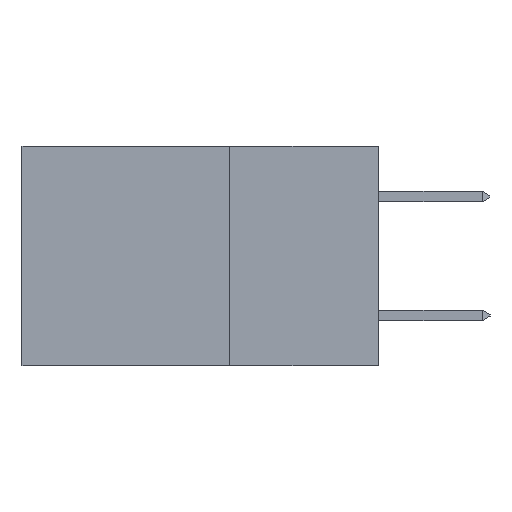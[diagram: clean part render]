
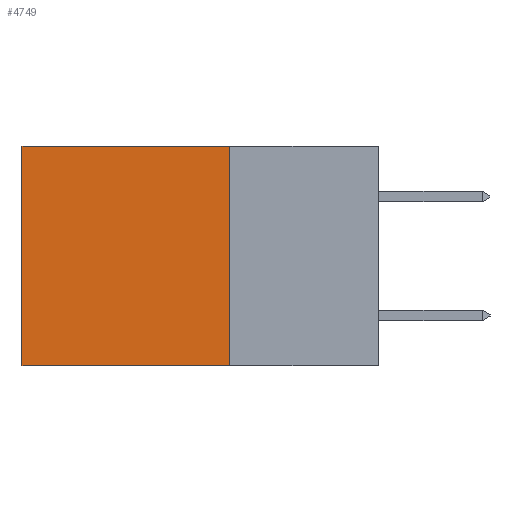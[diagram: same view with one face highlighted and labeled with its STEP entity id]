
A CAD part, left-side view. The second image highlights one B-rep face of the part: STEP entity #4749.
In plain terms, the highlighted planar face has unit normal (-1, 0, 0).
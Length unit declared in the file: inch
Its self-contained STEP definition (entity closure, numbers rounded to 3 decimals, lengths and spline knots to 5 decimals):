
#139 = DIRECTION ( 'NONE',  ( 0., 1., 0. ) ) ;
#163 = CARTESIAN_POINT ( 'NONE',  ( 0.2615, 0.25, -0.37 ) ) ;
#863 = EDGE_CURVE ( 'NONE', #10106, #3517, #16603, .T. ) ;
#1203 = VERTEX_POINT ( 'NONE', #9396 ) ;
#1410 = LINE ( 'NONE', #14508, #16244 ) ;
#3517 = VERTEX_POINT ( 'NONE', #10475 ) ;
#3588 = ORIENTED_EDGE ( 'NONE', *, *, #12488, .T. ) ;
#3818 = CARTESIAN_POINT ( 'NONE',  ( 0.2615, 0.25, 0. ) ) ;
#4409 = EDGE_CURVE ( 'NONE', #3517, #15597, #15761, .T. ) ;
#4731 = VECTOR ( 'NONE', #139, 39.37008 ) ;
#4749 = ADVANCED_FACE ( 'NONE', ( #17815 ), #11649, .F. ) ;
#5098 = EDGE_CURVE ( 'NONE', #10106, #1203, #12778, .T. ) ;
#5652 = VECTOR ( 'NONE', #16321, 39.37008 ) ;
#6225 = DIRECTION ( 'NONE',  ( 0., 0., -1. ) ) ;
#6708 = DIRECTION ( 'NONE',  ( 0., 1., 0. ) ) ;
#9093 = VECTOR ( 'NONE', #6708, 39.37008 ) ;
#9396 = CARTESIAN_POINT ( 'NONE',  ( 0.2615, 0.6, 0. ) ) ;
#9405 = AXIS2_PLACEMENT_3D ( 'NONE', #11943, #11572, #11391 ) ;
#10106 = VERTEX_POINT ( 'NONE', #16556 ) ;
#10475 = CARTESIAN_POINT ( 'NONE',  ( 0.2615, 0.25, -0.37 ) ) ;
#11391 = DIRECTION ( 'NONE',  ( 0., 0., -1. ) ) ;
#11572 = DIRECTION ( 'NONE',  ( 1., 0., 0. ) ) ;
#11649 = PLANE ( 'NONE',  #9405 ) ;
#11943 = CARTESIAN_POINT ( 'NONE',  ( 0.2615, 0.25, -0.37 ) ) ;
#12365 = ORIENTED_EDGE ( 'NONE', *, *, #863, .F. ) ;
#12488 = EDGE_CURVE ( 'NONE', #1203, #15597, #1410, .T. ) ;
#12778 = LINE ( 'NONE', #3818, #9093 ) ;
#12897 = ORIENTED_EDGE ( 'NONE', *, *, #4409, .F. ) ;
#13500 = ORIENTED_EDGE ( 'NONE', *, *, #5098, .T. ) ;
#14176 = CARTESIAN_POINT ( 'NONE',  ( 0.2615, 0.6, -0.37 ) ) ;
#14508 = CARTESIAN_POINT ( 'NONE',  ( 0.2615, 0.6, -0.37 ) ) ;
#15597 = VERTEX_POINT ( 'NONE', #14176 ) ;
#15659 = EDGE_LOOP ( 'NONE', ( #3588, #12897, #12365, #13500 ) ) ;
#15761 = LINE ( 'NONE', #163, #4731 ) ;
#16244 = VECTOR ( 'NONE', #6225, 39.37008 ) ;
#16321 = DIRECTION ( 'NONE',  ( 0., 0., -1. ) ) ;
#16556 = CARTESIAN_POINT ( 'NONE',  ( 0.2615, 0.25, 0. ) ) ;
#16603 = LINE ( 'NONE', #17102, #5652 ) ;
#17102 = CARTESIAN_POINT ( 'NONE',  ( 0.2615, 0.25, -0.37 ) ) ;
#17815 = FACE_OUTER_BOUND ( 'NONE', #15659, .T. ) ;
